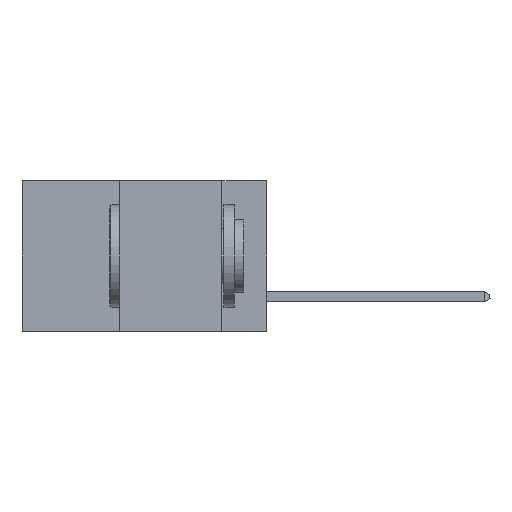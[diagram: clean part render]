
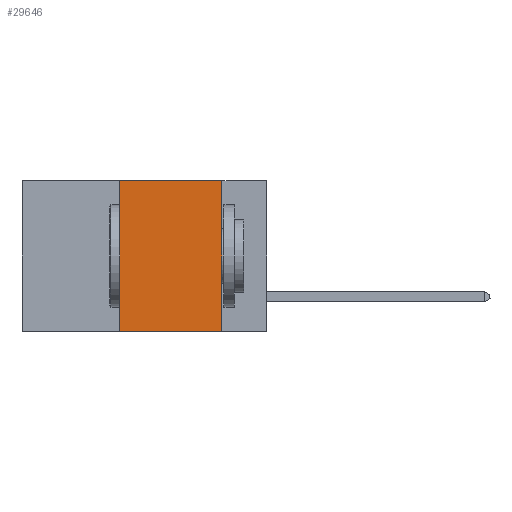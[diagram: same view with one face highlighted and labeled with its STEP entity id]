
A CAD part, left-side view. The second image highlights one B-rep face of the part: STEP entity #29646.
In plain terms, the highlighted planar face has unit normal (-1, 0, 0).
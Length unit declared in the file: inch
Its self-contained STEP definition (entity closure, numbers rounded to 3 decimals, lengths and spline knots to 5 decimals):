
#866 = EDGE_CURVE ( 'NONE', #22895, #20394, #29585, .T. ) ;
#1712 = VECTOR ( 'NONE', #11200, 39.37008 ) ;
#2177 = CARTESIAN_POINT ( 'NONE',  ( 0., 0.36, 0. ) ) ;
#2736 = AXIS2_PLACEMENT_3D ( 'NONE', #13855, #3502, #11352 ) ;
#3502 = DIRECTION ( 'NONE',  ( 1., 0., 0. ) ) ;
#4465 = VERTEX_POINT ( 'NONE', #6506 ) ;
#4567 = ORIENTED_EDGE ( 'NONE', *, *, #26432, .F. ) ;
#6506 = CARTESIAN_POINT ( 'NONE',  ( 0., 0.36, -0.37 ) ) ;
#6644 = LINE ( 'NONE', #14212, #29811 ) ;
#6742 = DIRECTION ( 'NONE',  ( 0., 0., -1. ) ) ;
#7095 = ORIENTED_EDGE ( 'NONE', *, *, #866, .F. ) ;
#7117 = VERTEX_POINT ( 'NONE', #2177 ) ;
#9318 = ORIENTED_EDGE ( 'NONE', *, *, #26588, .T. ) ;
#9486 = LINE ( 'NONE', #20204, #11100 ) ;
#11100 = VECTOR ( 'NONE', #33246, 39.37008 ) ;
#11200 = DIRECTION ( 'NONE',  ( 0., -1., 0. ) ) ;
#11352 = DIRECTION ( 'NONE',  ( 0., 0., -1. ) ) ;
#11482 = EDGE_LOOP ( 'NONE', ( #7095, #4567, #31118, #9318 ) ) ;
#13855 = CARTESIAN_POINT ( 'NONE',  ( 0., 0.6, 0. ) ) ;
#14212 = CARTESIAN_POINT ( 'NONE',  ( 0., 0.36, 0. ) ) ;
#15170 = LINE ( 'NONE', #31488, #1712 ) ;
#15350 = CARTESIAN_POINT ( 'NONE',  ( 0., 0.11, -0.37 ) ) ;
#20204 = CARTESIAN_POINT ( 'NONE',  ( 0., 0.6, 0. ) ) ;
#20394 = VERTEX_POINT ( 'NONE', #15350 ) ;
#20972 = EDGE_CURVE ( 'NONE', #4465, #7117, #6644, .T. ) ;
#21536 = PLANE ( 'NONE',  #2736 ) ;
#22639 = CARTESIAN_POINT ( 'NONE',  ( 0., 0.11, 0. ) ) ;
#22895 = VERTEX_POINT ( 'NONE', #26889 ) ;
#23756 = FACE_OUTER_BOUND ( 'NONE', #11482, .T. ) ;
#24618 = DIRECTION ( 'NONE',  ( 0., 0., 1. ) ) ;
#26432 = EDGE_CURVE ( 'NONE', #7117, #22895, #9486, .T. ) ;
#26588 = EDGE_CURVE ( 'NONE', #4465, #20394, #15170, .T. ) ;
#26889 = CARTESIAN_POINT ( 'NONE',  ( 0., 0.11, 0. ) ) ;
#29585 = LINE ( 'NONE', #22639, #31582 ) ;
#29646 = ADVANCED_FACE ( 'NONE', ( #23756 ), #21536, .F. ) ;
#29811 = VECTOR ( 'NONE', #24618, 39.37008 ) ;
#31118 = ORIENTED_EDGE ( 'NONE', *, *, #20972, .F. ) ;
#31488 = CARTESIAN_POINT ( 'NONE',  ( 0., 0.6, -0.37 ) ) ;
#31582 = VECTOR ( 'NONE', #6742, 39.37008 ) ;
#33246 = DIRECTION ( 'NONE',  ( 0., -1., 0. ) ) ;
